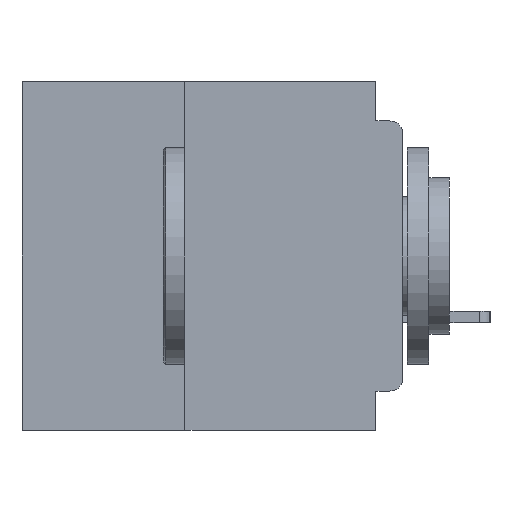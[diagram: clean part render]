
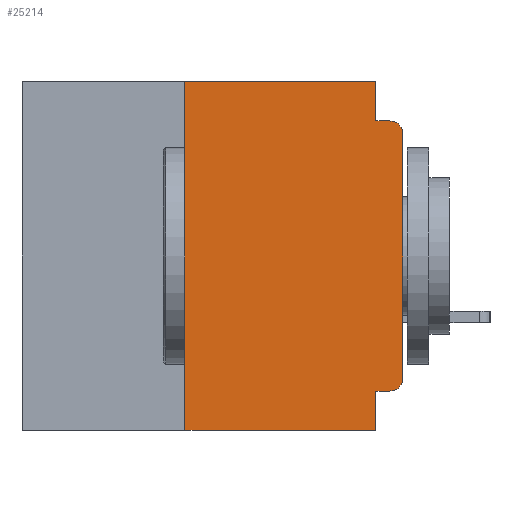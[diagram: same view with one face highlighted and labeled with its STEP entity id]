
A CAD part, left-side view. The second image highlights one B-rep face of the part: STEP entity #25214.
In plain terms, the highlighted planar face has unit normal (-1, 0, 0).
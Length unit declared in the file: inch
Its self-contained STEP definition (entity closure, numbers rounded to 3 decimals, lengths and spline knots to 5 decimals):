
#336 = EDGE_CURVE ( 'NONE', #7256, #5254, #5537, .T. ) ;
#783 = EDGE_CURVE ( 'NONE', #26726, #15129, #5500, .T. ) ;
#988 = VERTEX_POINT ( 'NONE', #21764 ) ;
#1404 = DIRECTION ( 'NONE',  ( 0., -1., 0. ) ) ;
#1908 = FACE_OUTER_BOUND ( 'NONE', #19538, .T. ) ;
#2462 = ORIENTED_EDGE ( 'NONE', *, *, #27691, .T. ) ;
#3016 = LINE ( 'NONE', #38887, #39941 ) ;
#3091 = ORIENTED_EDGE ( 'NONE', *, *, #15165, .F. ) ;
#4002 = LINE ( 'NONE', #22096, #12392 ) ;
#4087 = ORIENTED_EDGE ( 'NONE', *, *, #43958, .F. ) ;
#4167 = LINE ( 'NONE', #8622, #41082 ) ;
#5196 = PLANE ( 'NONE',  #37228 ) ;
#5254 = VERTEX_POINT ( 'NONE', #36560 ) ;
#5500 = CIRCLE ( 'NONE', #41980, 0.015 ) ;
#5537 = LINE ( 'NONE', #29174, #31825 ) ;
#6410 = LINE ( 'NONE', #30007, #43338 ) ;
#7256 = VERTEX_POINT ( 'NONE', #44875 ) ;
#8038 = ORIENTED_EDGE ( 'NONE', *, *, #9476, .F. ) ;
#8622 = CARTESIAN_POINT ( 'NONE',  ( 0., 0., -0.045 ) ) ;
#8792 = DIRECTION ( 'NONE',  ( 0., 0., -1. ) ) ;
#9476 = EDGE_CURVE ( 'NONE', #38720, #15129, #4167, .T. ) ;
#9668 = VERTEX_POINT ( 'NONE', #41890 ) ;
#10449 = VECTOR ( 'NONE', #27664, 39.37008 ) ;
#11584 = DIRECTION ( 'NONE',  ( -1., 0., 0. ) ) ;
#11880 = ORIENTED_EDGE ( 'NONE', *, *, #41104, .F. ) ;
#12392 = VECTOR ( 'NONE', #25685, 39.37008 ) ;
#15129 = VERTEX_POINT ( 'NONE', #24064 ) ;
#15165 = EDGE_CURVE ( 'NONE', #28237, #9668, #29420, .T. ) ;
#16622 = DIRECTION ( 'NONE',  ( 0., 0., -1. ) ) ;
#16708 = DIRECTION ( 'NONE',  ( 0., 0., 1. ) ) ;
#17017 = DIRECTION ( 'NONE',  ( 0., 0., -1. ) ) ;
#17070 = CARTESIAN_POINT ( 'NONE',  ( 0., 0., -0.355 ) ) ;
#17461 = DIRECTION ( 'NONE',  ( 0., 0., 1. ) ) ;
#19538 = EDGE_LOOP ( 'NONE', ( #2462, #32602, #8038, #11880, #4087, #29213, #21876, #28835, #3091, #20064 ) ) ;
#19569 = VECTOR ( 'NONE', #16708, 39.37008 ) ;
#20064 = ORIENTED_EDGE ( 'NONE', *, *, #30417, .T. ) ;
#20476 = VERTEX_POINT ( 'NONE', #26503 ) ;
#20567 = CARTESIAN_POINT ( 'NONE',  ( 0., 0., 0. ) ) ;
#21764 = CARTESIAN_POINT ( 'NONE',  ( 0., 0., -0.34 ) ) ;
#21876 = ORIENTED_EDGE ( 'NONE', *, *, #336, .T. ) ;
#22096 = CARTESIAN_POINT ( 'NONE',  ( 0., 0.031, -0.4 ) ) ;
#22939 = CARTESIAN_POINT ( 'NONE',  ( 0., 0.437, 0. ) ) ;
#24064 = CARTESIAN_POINT ( 'NONE',  ( 0., 0.015, -0.045 ) ) ;
#24742 = CARTESIAN_POINT ( 'NONE',  ( 0., 0.015, -0.06 ) ) ;
#24936 = DIRECTION ( 'NONE',  ( -1., 0., 0. ) ) ;
#25214 = ADVANCED_FACE ( 'NONE', ( #1908 ), #5196, .F. ) ;
#25685 = DIRECTION ( 'NONE',  ( 0., 0., -1. ) ) ;
#26503 = CARTESIAN_POINT ( 'NONE',  ( 0., 0.25, 0. ) ) ;
#26726 = VERTEX_POINT ( 'NONE', #39473 ) ;
#27299 = DIRECTION ( 'NONE',  ( 0., -1., 0. ) ) ;
#27664 = DIRECTION ( 'NONE',  ( 0., 1., 0. ) ) ;
#27691 = EDGE_CURVE ( 'NONE', #988, #26726, #38642, .T. ) ;
#28237 = VERTEX_POINT ( 'NONE', #45122 ) ;
#28349 = AXIS2_PLACEMENT_3D ( 'NONE', #32969, #11584, #36557 ) ;
#28835 = ORIENTED_EDGE ( 'NONE', *, *, #34746, .F. ) ;
#29138 = DIRECTION ( 'NONE',  ( 0., -1., 0. ) ) ;
#29174 = CARTESIAN_POINT ( 'NONE',  ( 0., 0.437, -0.4 ) ) ;
#29213 = ORIENTED_EDGE ( 'NONE', *, *, #36265, .F. ) ;
#29420 = LINE ( 'NONE', #17070, #10449 ) ;
#30007 = CARTESIAN_POINT ( 'NONE',  ( 0., 0.437, 0. ) ) ;
#30015 = VERTEX_POINT ( 'NONE', #33760 ) ;
#30182 = DIRECTION ( 'NONE',  ( 1., 0., 0. ) ) ;
#30417 = EDGE_CURVE ( 'NONE', #28237, #988, #34519, .T. ) ;
#30558 = LINE ( 'NONE', #41691, #38945 ) ;
#31825 = VECTOR ( 'NONE', #29138, 39.37008 ) ;
#32602 = ORIENTED_EDGE ( 'NONE', *, *, #783, .T. ) ;
#32969 = CARTESIAN_POINT ( 'NONE',  ( 0., 0.015, -0.34 ) ) ;
#33760 = CARTESIAN_POINT ( 'NONE',  ( 0., 0.031, 0. ) ) ;
#34519 = CIRCLE ( 'NONE', #28349, 0.015 ) ;
#34746 = EDGE_CURVE ( 'NONE', #9668, #5254, #4002, .T. ) ;
#36265 = EDGE_CURVE ( 'NONE', #7256, #20476, #3016, .T. ) ;
#36557 = DIRECTION ( 'NONE',  ( 0., 0., -1. ) ) ;
#36560 = CARTESIAN_POINT ( 'NONE',  ( 0., 0.031, -0.4 ) ) ;
#37228 = AXIS2_PLACEMENT_3D ( 'NONE', #22939, #30182, #8792 ) ;
#38116 = CARTESIAN_POINT ( 'NONE',  ( 0., 0.031, -0.045 ) ) ;
#38642 = LINE ( 'NONE', #20567, #19569 ) ;
#38720 = VERTEX_POINT ( 'NONE', #38116 ) ;
#38887 = CARTESIAN_POINT ( 'NONE',  ( 0., 0.25, -0.4 ) ) ;
#38945 = VECTOR ( 'NONE', #16622, 39.37008 ) ;
#39473 = CARTESIAN_POINT ( 'NONE',  ( 0., 0., -0.06 ) ) ;
#39941 = VECTOR ( 'NONE', #17461, 39.37008 ) ;
#41082 = VECTOR ( 'NONE', #1404, 39.37008 ) ;
#41104 = EDGE_CURVE ( 'NONE', #30015, #38720, #30558, .T. ) ;
#41691 = CARTESIAN_POINT ( 'NONE',  ( 0., 0.031, 0. ) ) ;
#41890 = CARTESIAN_POINT ( 'NONE',  ( 0., 0.031, -0.355 ) ) ;
#41980 = AXIS2_PLACEMENT_3D ( 'NONE', #24742, #24936, #17017 ) ;
#43338 = VECTOR ( 'NONE', #27299, 39.37008 ) ;
#43958 = EDGE_CURVE ( 'NONE', #20476, #30015, #6410, .T. ) ;
#44875 = CARTESIAN_POINT ( 'NONE',  ( 0., 0.25, -0.4 ) ) ;
#45122 = CARTESIAN_POINT ( 'NONE',  ( 0., 0.015, -0.355 ) ) ;
